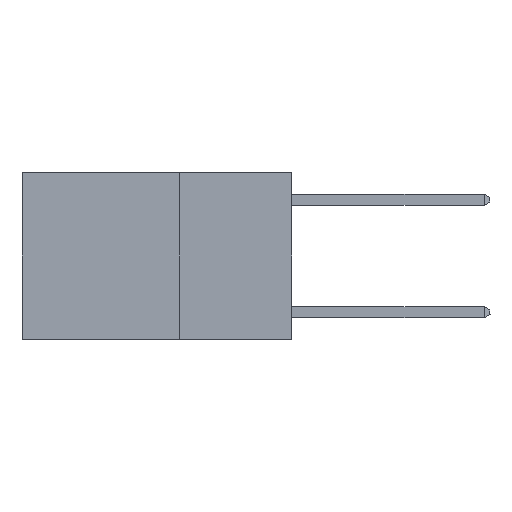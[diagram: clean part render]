
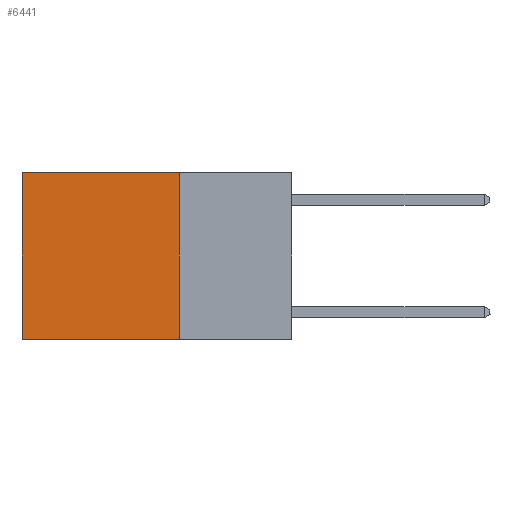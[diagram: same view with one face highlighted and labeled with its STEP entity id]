
A CAD part, left-side view. The second image highlights one B-rep face of the part: STEP entity #6441.
In plain terms, the highlighted planar face has unit normal (-1, 0, 0).
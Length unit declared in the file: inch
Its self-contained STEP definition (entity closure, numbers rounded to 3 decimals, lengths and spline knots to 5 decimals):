
#516 = LINE ( 'NONE', #11988, #5619 ) ;
#917 = LINE ( 'NONE', #9560, #5343 ) ;
#949 = DIRECTION ( 'NONE',  ( 1., 0., 0. ) ) ;
#1434 = CARTESIAN_POINT ( 'NONE',  ( 0.2625, 0.25, 0. ) ) ;
#2939 = CARTESIAN_POINT ( 'NONE',  ( 0.2625, 0.25, -0.37 ) ) ;
#3023 = LINE ( 'NONE', #1434, #8072 ) ;
#3497 = DIRECTION ( 'NONE',  ( 0., 0., -1. ) ) ;
#3986 = EDGE_CURVE ( 'NONE', #10012, #9996, #917, .T. ) ;
#4496 = LINE ( 'NONE', #5110, #9498 ) ;
#4723 = ORIENTED_EDGE ( 'NONE', *, *, #8365, .F. ) ;
#4908 = ORIENTED_EDGE ( 'NONE', *, *, #3986, .T. ) ;
#5110 = CARTESIAN_POINT ( 'NONE',  ( 0.2625, 0.25, 0. ) ) ;
#5256 = ORIENTED_EDGE ( 'NONE', *, *, #10752, .T. ) ;
#5324 = ORIENTED_EDGE ( 'NONE', *, *, #5328, .F. ) ;
#5328 = EDGE_CURVE ( 'NONE', #8641, #5657, #3023, .T. ) ;
#5343 = VECTOR ( 'NONE', #8624, 39.37008 ) ;
#5619 = VECTOR ( 'NONE', #10067, 39.37008 ) ;
#5657 = VERTEX_POINT ( 'NONE', #2939 ) ;
#6441 = ADVANCED_FACE ( 'NONE', ( #10407 ), #9955, .F. ) ;
#7025 = CARTESIAN_POINT ( 'NONE',  ( 0.2625, 0.25, 0. ) ) ;
#7805 = EDGE_LOOP ( 'NONE', ( #4908, #4723, #5324, #5256 ) ) ;
#8072 = VECTOR ( 'NONE', #3497, 39.37008 ) ;
#8099 = DIRECTION ( 'NONE',  ( 0., 0., -1. ) ) ;
#8365 = EDGE_CURVE ( 'NONE', #5657, #9996, #516, .T. ) ;
#8624 = DIRECTION ( 'NONE',  ( 0., 0., -1. ) ) ;
#8641 = VERTEX_POINT ( 'NONE', #10394 ) ;
#9059 = CARTESIAN_POINT ( 'NONE',  ( 0.2625, 0.6, 0. ) ) ;
#9498 = VECTOR ( 'NONE', #11052, 39.37008 ) ;
#9560 = CARTESIAN_POINT ( 'NONE',  ( 0.2625, 0.6, 0. ) ) ;
#9955 = PLANE ( 'NONE',  #12682 ) ;
#9996 = VERTEX_POINT ( 'NONE', #12861 ) ;
#10012 = VERTEX_POINT ( 'NONE', #9059 ) ;
#10067 = DIRECTION ( 'NONE',  ( 0., 1., 0. ) ) ;
#10394 = CARTESIAN_POINT ( 'NONE',  ( 0.2625, 0.25, 0. ) ) ;
#10407 = FACE_OUTER_BOUND ( 'NONE', #7805, .T. ) ;
#10752 = EDGE_CURVE ( 'NONE', #8641, #10012, #4496, .T. ) ;
#11052 = DIRECTION ( 'NONE',  ( 0., 1., 0. ) ) ;
#11988 = CARTESIAN_POINT ( 'NONE',  ( 0.2625, 0.25, -0.37 ) ) ;
#12682 = AXIS2_PLACEMENT_3D ( 'NONE', #7025, #949, #8099 ) ;
#12861 = CARTESIAN_POINT ( 'NONE',  ( 0.2625, 0.6, -0.37 ) ) ;
